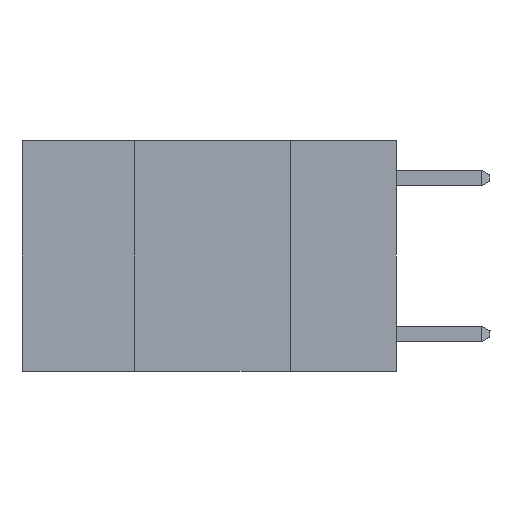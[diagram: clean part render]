
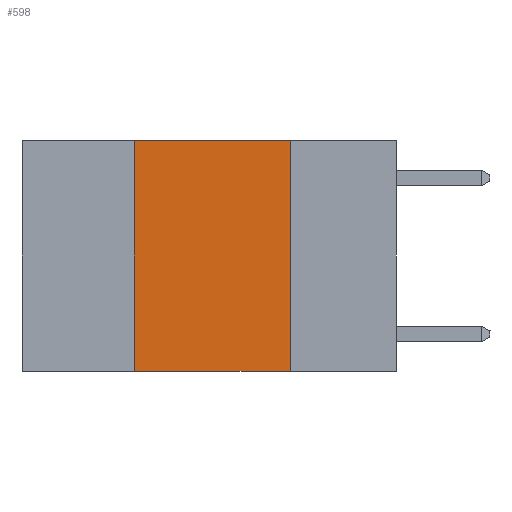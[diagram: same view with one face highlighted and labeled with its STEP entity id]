
A CAD part, left-side view. The second image highlights one B-rep face of the part: STEP entity #598.
In plain terms, the highlighted planar face has unit normal (-1, 0, 0).
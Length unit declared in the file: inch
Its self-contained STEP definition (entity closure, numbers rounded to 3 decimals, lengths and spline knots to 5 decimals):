
#598 = ADVANCED_FACE ( 'NONE', ( #14497 ), #3370, .F. ) ;
#857 = VECTOR ( 'NONE', #11085, 39.37008 ) ;
#1404 = AXIS2_PLACEMENT_3D ( 'NONE', #4867, #15099, #16141 ) ;
#1514 = ORIENTED_EDGE ( 'NONE', *, *, #10039, .T. ) ;
#2255 = ORIENTED_EDGE ( 'NONE', *, *, #8286, .F. ) ;
#2805 = ORIENTED_EDGE ( 'NONE', *, *, #6883, .F. ) ;
#2873 = VERTEX_POINT ( 'NONE', #5175 ) ;
#3277 = CARTESIAN_POINT ( 'NONE',  ( 0., 0.6, -0.37 ) ) ;
#3345 = VECTOR ( 'NONE', #15083, 39.37008 ) ;
#3370 = PLANE ( 'NONE',  #1404 ) ;
#3850 = LINE ( 'NONE', #3277, #14197 ) ;
#4664 = DIRECTION ( 'NONE',  ( 0., -1., 0. ) ) ;
#4867 = CARTESIAN_POINT ( 'NONE',  ( 0., 0.6, 0. ) ) ;
#4941 = CARTESIAN_POINT ( 'NONE',  ( 0., 0.42, 0. ) ) ;
#5175 = CARTESIAN_POINT ( 'NONE',  ( 0., 0.17, 0. ) ) ;
#5196 = ORIENTED_EDGE ( 'NONE', *, *, #11597, .F. ) ;
#6883 = EDGE_CURVE ( 'NONE', #15034, #2873, #16733, .T. ) ;
#7353 = VERTEX_POINT ( 'NONE', #10533 ) ;
#8042 = LINE ( 'NONE', #9756, #857 ) ;
#8286 = EDGE_CURVE ( 'NONE', #2873, #16425, #8042, .T. ) ;
#9496 = EDGE_LOOP ( 'NONE', ( #2255, #2805, #5196, #1514 ) ) ;
#9756 = CARTESIAN_POINT ( 'NONE',  ( 0., 0.17, 0. ) ) ;
#10039 = EDGE_CURVE ( 'NONE', #7353, #16425, #3850, .T. ) ;
#10138 = VECTOR ( 'NONE', #11947, 39.37008 ) ;
#10533 = CARTESIAN_POINT ( 'NONE',  ( 0., 0.42, -0.37 ) ) ;
#11079 = CARTESIAN_POINT ( 'NONE',  ( 0., 0.42, 0. ) ) ;
#11085 = DIRECTION ( 'NONE',  ( 0., 0., -1. ) ) ;
#11597 = EDGE_CURVE ( 'NONE', #7353, #15034, #14125, .T. ) ;
#11947 = DIRECTION ( 'NONE',  ( 0., -1., 0. ) ) ;
#12510 = CARTESIAN_POINT ( 'NONE',  ( 0., 0.17, -0.37 ) ) ;
#14125 = LINE ( 'NONE', #11079, #3345 ) ;
#14197 = VECTOR ( 'NONE', #4664, 39.37008 ) ;
#14497 = FACE_OUTER_BOUND ( 'NONE', #9496, .T. ) ;
#14614 = CARTESIAN_POINT ( 'NONE',  ( 0., 0.6, 0. ) ) ;
#15034 = VERTEX_POINT ( 'NONE', #4941 ) ;
#15083 = DIRECTION ( 'NONE',  ( 0., 0., 1. ) ) ;
#15099 = DIRECTION ( 'NONE',  ( 1., 0., 0. ) ) ;
#16141 = DIRECTION ( 'NONE',  ( 0., 0., -1. ) ) ;
#16425 = VERTEX_POINT ( 'NONE', #12510 ) ;
#16733 = LINE ( 'NONE', #14614, #10138 ) ;
